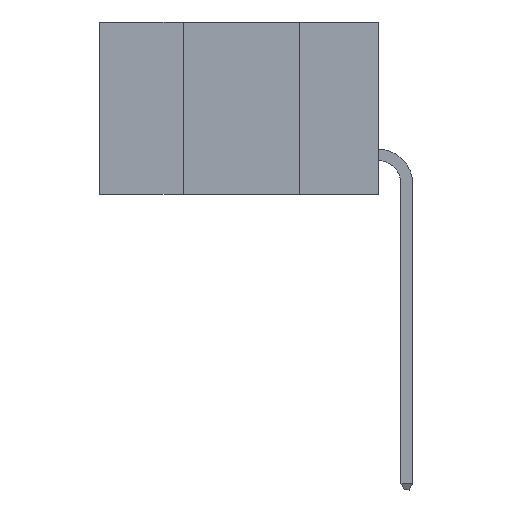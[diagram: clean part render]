
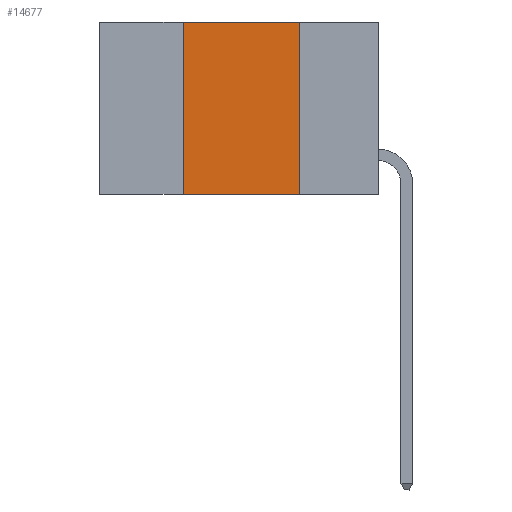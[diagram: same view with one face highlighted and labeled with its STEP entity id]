
A CAD part, left-side view. The second image highlights one B-rep face of the part: STEP entity #14677.
In plain terms, the highlighted planar face has unit normal (-1, 0, 0).
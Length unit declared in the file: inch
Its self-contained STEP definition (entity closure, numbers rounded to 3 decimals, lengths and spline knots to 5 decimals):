
#318 = VERTEX_POINT ( 'NONE', #13621 ) ;
#373 = CARTESIAN_POINT ( 'NONE',  ( 0., 0.42, 0. ) ) ;
#2040 = ORIENTED_EDGE ( 'NONE', *, *, #8210, .F. ) ;
#2475 = DIRECTION ( 'NONE',  ( 0., 0., -1. ) ) ;
#2539 = PLANE ( 'NONE',  #14798 ) ;
#2769 = ORIENTED_EDGE ( 'NONE', *, *, #16586, .F. ) ;
#3403 = LINE ( 'NONE', #20039, #23105 ) ;
#3616 = ORIENTED_EDGE ( 'NONE', *, *, #17094, .F. ) ;
#3654 = VERTEX_POINT ( 'NONE', #16922 ) ;
#3936 = DIRECTION ( 'NONE',  ( 0., 0., 1. ) ) ;
#4659 = LINE ( 'NONE', #12885, #24393 ) ;
#4690 = DIRECTION ( 'NONE',  ( 1., 0., 0. ) ) ;
#6857 = EDGE_CURVE ( 'NONE', #8966, #318, #4659, .T. ) ;
#7058 = DIRECTION ( 'NONE',  ( 0., -1., 0. ) ) ;
#7221 = CARTESIAN_POINT ( 'NONE',  ( 0., 0.42, 0. ) ) ;
#8210 = EDGE_CURVE ( 'NONE', #8966, #20639, #13420, .T. ) ;
#8966 = VERTEX_POINT ( 'NONE', #20484 ) ;
#10372 = ORIENTED_EDGE ( 'NONE', *, *, #6857, .T. ) ;
#10693 = DIRECTION ( 'NONE',  ( 0., -1., 0. ) ) ;
#11451 = EDGE_LOOP ( 'NONE', ( #3616, #2769, #2040, #10372 ) ) ;
#12545 = DIRECTION ( 'NONE',  ( 0., 0., -1. ) ) ;
#12885 = CARTESIAN_POINT ( 'NONE',  ( 0., 0.6, -0.37 ) ) ;
#13420 = LINE ( 'NONE', #373, #20574 ) ;
#13621 = CARTESIAN_POINT ( 'NONE',  ( 0., 0.17, -0.37 ) ) ;
#14457 = VECTOR ( 'NONE', #2475, 39.37008 ) ;
#14677 = ADVANCED_FACE ( 'NONE', ( #20525 ), #2539, .F. ) ;
#14798 = AXIS2_PLACEMENT_3D ( 'NONE', #15920, #4690, #12545 ) ;
#15086 = LINE ( 'NONE', #16197, #14457 ) ;
#15920 = CARTESIAN_POINT ( 'NONE',  ( 0., 0.6, 0. ) ) ;
#16197 = CARTESIAN_POINT ( 'NONE',  ( 0., 0.17, 0. ) ) ;
#16586 = EDGE_CURVE ( 'NONE', #20639, #3654, #3403, .T. ) ;
#16922 = CARTESIAN_POINT ( 'NONE',  ( 0., 0.17, 0. ) ) ;
#17094 = EDGE_CURVE ( 'NONE', #3654, #318, #15086, .T. ) ;
#20039 = CARTESIAN_POINT ( 'NONE',  ( 0., 0.6, 0. ) ) ;
#20484 = CARTESIAN_POINT ( 'NONE',  ( 0., 0.42, -0.37 ) ) ;
#20525 = FACE_OUTER_BOUND ( 'NONE', #11451, .T. ) ;
#20574 = VECTOR ( 'NONE', #3936, 39.37008 ) ;
#20639 = VERTEX_POINT ( 'NONE', #7221 ) ;
#23105 = VECTOR ( 'NONE', #10693, 39.37008 ) ;
#24393 = VECTOR ( 'NONE', #7058, 39.37008 ) ;
